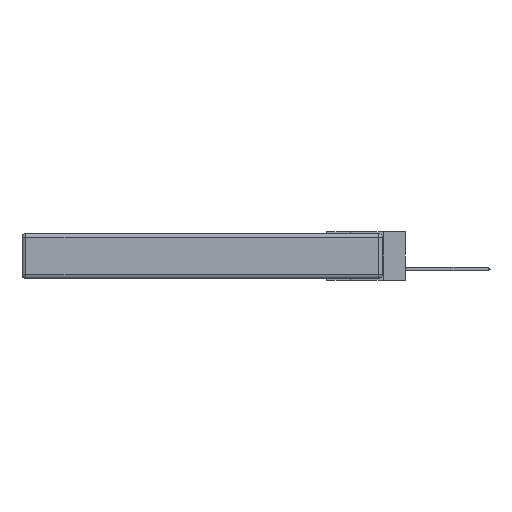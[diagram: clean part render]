
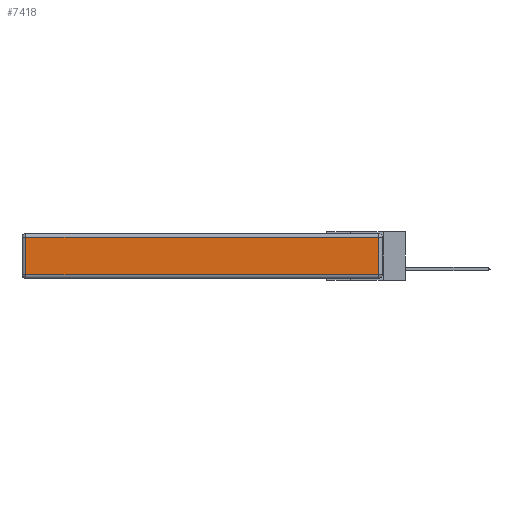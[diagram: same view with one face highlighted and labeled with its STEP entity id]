
A CAD part, left-side view. The second image highlights one B-rep face of the part: STEP entity #7418.
In plain terms, the highlighted planar face has unit normal (-1, 0, 0).
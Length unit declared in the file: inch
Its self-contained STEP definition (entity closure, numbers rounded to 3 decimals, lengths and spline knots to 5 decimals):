
#643 = ORIENTED_EDGE ( 'NONE', *, *, #10322, .T. ) ;
#688 = DIRECTION ( 'NONE',  ( 0., -1., 0. ) ) ;
#1160 = ORIENTED_EDGE ( 'NONE', *, *, #10806, .T. ) ;
#1299 = CARTESIAN_POINT ( 'NONE',  ( 0., 2.72, -0.313 ) ) ;
#1309 = VECTOR ( 'NONE', #688, 39.37008 ) ;
#1421 = VECTOR ( 'NONE', #5808, 39.37008 ) ;
#1745 = VECTOR ( 'NONE', #6227, 39.37008 ) ;
#2617 = CARTESIAN_POINT ( 'NONE',  ( 0., 2.75, -0.03 ) ) ;
#2862 = LINE ( 'NONE', #4781, #1421 ) ;
#2903 = VERTEX_POINT ( 'NONE', #1299 ) ;
#4181 = EDGE_CURVE ( 'NONE', #6212, #8192, #8110, .T. ) ;
#4775 = CARTESIAN_POINT ( 'NONE',  ( 0., 0., -0.343 ) ) ;
#4781 = CARTESIAN_POINT ( 'NONE',  ( 0., 2.72, -0.343 ) ) ;
#4927 = ORIENTED_EDGE ( 'NONE', *, *, #11861, .T. ) ;
#5551 = AXIS2_PLACEMENT_3D ( 'NONE', #4775, #11286, #5716 ) ;
#5716 = DIRECTION ( 'NONE',  ( 0., 0., 1. ) ) ;
#5808 = DIRECTION ( 'NONE',  ( 0., 0., -1. ) ) ;
#5864 = FACE_OUTER_BOUND ( 'NONE', #10732, .T. ) ;
#5987 = ORIENTED_EDGE ( 'NONE', *, *, #4181, .T. ) ;
#6212 = VERTEX_POINT ( 'NONE', #6981 ) ;
#6227 = DIRECTION ( 'NONE',  ( 0., 0., 1. ) ) ;
#6779 = PLANE ( 'NONE',  #5551 ) ;
#6966 = CARTESIAN_POINT ( 'NONE',  ( 0., 0.03, -0.313 ) ) ;
#6972 = VERTEX_POINT ( 'NONE', #6966 ) ;
#6981 = CARTESIAN_POINT ( 'NONE',  ( 0., 0.03, -0.03 ) ) ;
#7418 = ADVANCED_FACE ( 'NONE', ( #5864 ), #6779, .T. ) ;
#7569 = LINE ( 'NONE', #8017, #1309 ) ;
#8017 = CARTESIAN_POINT ( 'NONE',  ( 0., 0., -0.313 ) ) ;
#8110 = LINE ( 'NONE', #2617, #10304 ) ;
#8192 = VERTEX_POINT ( 'NONE', #10343 ) ;
#10304 = VECTOR ( 'NONE', #11950, 39.37008 ) ;
#10322 = EDGE_CURVE ( 'NONE', #6972, #6212, #11915, .T. ) ;
#10343 = CARTESIAN_POINT ( 'NONE',  ( 0., 2.72, -0.03 ) ) ;
#10732 = EDGE_LOOP ( 'NONE', ( #1160, #643, #5987, #4927 ) ) ;
#10806 = EDGE_CURVE ( 'NONE', #2903, #6972, #7569, .T. ) ;
#11286 = DIRECTION ( 'NONE',  ( -1., 0., 0. ) ) ;
#11795 = CARTESIAN_POINT ( 'NONE',  ( 0., 0.03, -0.343 ) ) ;
#11861 = EDGE_CURVE ( 'NONE', #8192, #2903, #2862, .T. ) ;
#11915 = LINE ( 'NONE', #11795, #1745 ) ;
#11950 = DIRECTION ( 'NONE',  ( 0., 1., 0. ) ) ;
